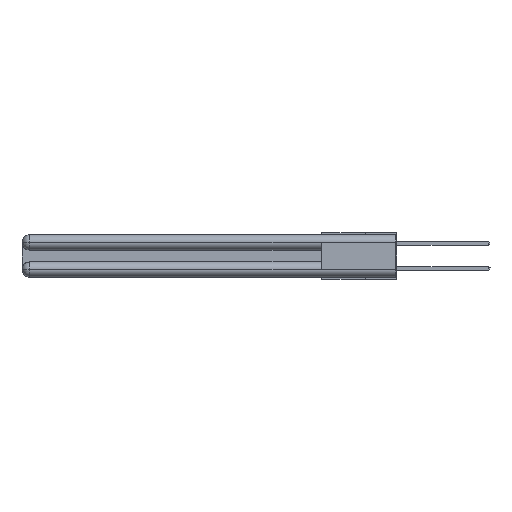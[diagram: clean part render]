
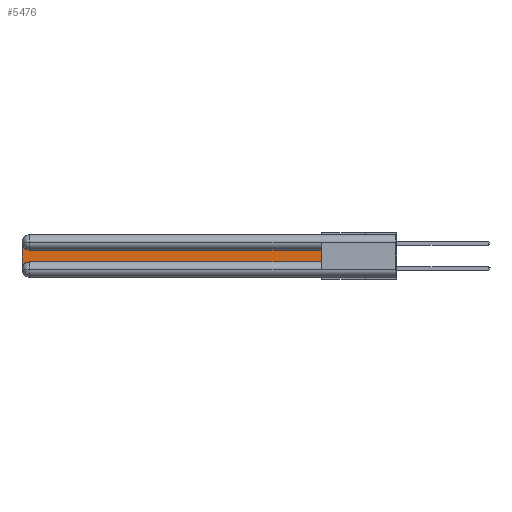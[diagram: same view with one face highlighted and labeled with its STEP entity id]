
A CAD part, left-side view. The second image highlights one B-rep face of the part: STEP entity #5476.
In plain terms, the highlighted planar face has unit normal (-1, 0, 0).
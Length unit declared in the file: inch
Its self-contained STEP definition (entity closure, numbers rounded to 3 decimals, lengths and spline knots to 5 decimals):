
#793 = CARTESIAN_POINT ( 'NONE',  ( 0.075, 0.6, -0.2175 ) ) ;
#1718 = LINE ( 'NONE', #13283, #29960 ) ;
#4207 = ORIENTED_EDGE ( 'NONE', *, *, #13217, .T. ) ;
#5051 = VECTOR ( 'NONE', #19397, 39.37008 ) ;
#5476 = ADVANCED_FACE ( 'NONE', ( #29121 ), #15105, .F. ) ;
#5946 = AXIS2_PLACEMENT_3D ( 'NONE', #17463, #17578, #22635 ) ;
#6285 = EDGE_CURVE ( 'NONE', #23076, #19812, #27012, .T. ) ;
#6788 = CIRCLE ( 'NONE', #29908, 0.06 ) ;
#7716 = LINE ( 'NONE', #16810, #18525 ) ;
#9128 = DIRECTION ( 'NONE',  ( 0., 0., -1. ) ) ;
#9418 = EDGE_CURVE ( 'NONE', #16564, #11968, #22975, .T. ) ;
#9884 = CARTESIAN_POINT ( 'NONE',  ( 0.075, 0.6, -0.2175 ) ) ;
#10523 = EDGE_CURVE ( 'NONE', #26097, #16564, #1718, .T. ) ;
#11637 = ORIENTED_EDGE ( 'NONE', *, *, #9418, .T. ) ;
#11968 = VERTEX_POINT ( 'NONE', #13987 ) ;
#13217 = EDGE_CURVE ( 'NONE', #19812, #26097, #34106, .T. ) ;
#13283 = CARTESIAN_POINT ( 'NONE',  ( 0.075, 0.6, -0.1225 ) ) ;
#13383 = VECTOR ( 'NONE', #17646, 39.37008 ) ;
#13987 = CARTESIAN_POINT ( 'NONE',  ( 0.075, 3., -0.0625 ) ) ;
#14328 = DIRECTION ( 'NONE',  ( 1., 0., 0. ) ) ;
#14566 = CARTESIAN_POINT ( 'NONE',  ( 0.075, 3., -0.2775 ) ) ;
#14990 = AXIS2_PLACEMENT_3D ( 'NONE', #20193, #22806, #25506 ) ;
#15105 = PLANE ( 'NONE',  #14990 ) ;
#16564 = VERTEX_POINT ( 'NONE', #17617 ) ;
#16810 = CARTESIAN_POINT ( 'NONE',  ( 0.075, 3., -0.2175 ) ) ;
#16881 = CARTESIAN_POINT ( 'NONE',  ( 0.075, 2.94, -0.2775 ) ) ;
#17463 = CARTESIAN_POINT ( 'NONE',  ( 0.075, 2.94, -0.0625 ) ) ;
#17578 = DIRECTION ( 'NONE',  ( 1., 0., 0. ) ) ;
#17617 = CARTESIAN_POINT ( 'NONE',  ( 0.075, 2.94, -0.1225 ) ) ;
#17646 = DIRECTION ( 'NONE',  ( 0., 0., 1. ) ) ;
#18525 = VECTOR ( 'NONE', #9128, 39.37008 ) ;
#18754 = DIRECTION ( 'NONE',  ( 0., 1., 0. ) ) ;
#19397 = DIRECTION ( 'NONE',  ( 0., -1., 0. ) ) ;
#19812 = VERTEX_POINT ( 'NONE', #24660 ) ;
#20193 = CARTESIAN_POINT ( 'NONE',  ( 0.075, 3., -0.1225 ) ) ;
#20791 = ORIENTED_EDGE ( 'NONE', *, *, #30356, .T. ) ;
#21326 = ORIENTED_EDGE ( 'NONE', *, *, #25670, .T. ) ;
#21949 = ORIENTED_EDGE ( 'NONE', *, *, #6285, .T. ) ;
#22635 = DIRECTION ( 'NONE',  ( 0., 0., -1. ) ) ;
#22806 = DIRECTION ( 'NONE',  ( 1., 0., 0. ) ) ;
#22975 = CIRCLE ( 'NONE', #5946, 0.06 ) ;
#23076 = VERTEX_POINT ( 'NONE', #30169 ) ;
#24660 = CARTESIAN_POINT ( 'NONE',  ( 0.075, 0.6, -0.2175 ) ) ;
#24844 = DIRECTION ( 'NONE',  ( 0., 0., -1. ) ) ;
#25506 = DIRECTION ( 'NONE',  ( 0., 0., -1. ) ) ;
#25670 = EDGE_CURVE ( 'NONE', #26879, #23076, #6788, .T. ) ;
#26097 = VERTEX_POINT ( 'NONE', #31408 ) ;
#26879 = VERTEX_POINT ( 'NONE', #14566 ) ;
#27012 = LINE ( 'NONE', #793, #5051 ) ;
#27372 = ORIENTED_EDGE ( 'NONE', *, *, #10523, .T. ) ;
#29121 = FACE_OUTER_BOUND ( 'NONE', #30140, .T. ) ;
#29908 = AXIS2_PLACEMENT_3D ( 'NONE', #16881, #14328, #24844 ) ;
#29960 = VECTOR ( 'NONE', #18754, 39.37008 ) ;
#30140 = EDGE_LOOP ( 'NONE', ( #27372, #11637, #20791, #21326, #21949, #4207 ) ) ;
#30169 = CARTESIAN_POINT ( 'NONE',  ( 0.075, 2.94, -0.2175 ) ) ;
#30356 = EDGE_CURVE ( 'NONE', #11968, #26879, #7716, .T. ) ;
#31408 = CARTESIAN_POINT ( 'NONE',  ( 0.075, 0.6, -0.1225 ) ) ;
#34106 = LINE ( 'NONE', #9884, #13383 ) ;
